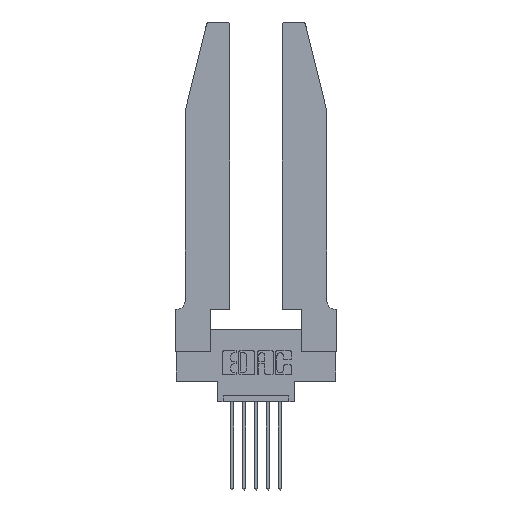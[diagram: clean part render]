
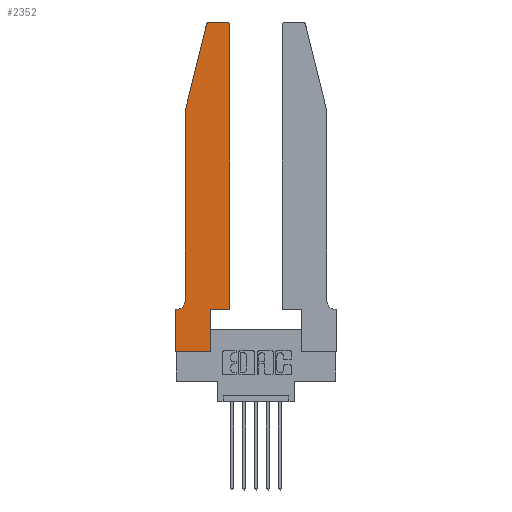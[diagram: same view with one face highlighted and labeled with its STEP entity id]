
A CAD part, top view. The second image highlights one B-rep face of the part: STEP entity #2352.
In plain terms, the highlighted planar face has unit normal (0, 0, 1).
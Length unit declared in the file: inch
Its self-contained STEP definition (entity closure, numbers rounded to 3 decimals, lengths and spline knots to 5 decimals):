
#86 = VERTEX_POINT ( 'NONE', #11882 ) ;
#117 = VECTOR ( 'NONE', #6942, 39.37008 ) ;
#277 = CARTESIAN_POINT ( 'NONE',  ( 0.284, 2.72, 0.37 ) ) ;
#532 = DIRECTION ( 'NONE',  ( 0., 1., 0. ) ) ;
#563 = VECTOR ( 'NONE', #11464, 39.37008 ) ;
#651 = EDGE_CURVE ( 'NONE', #5297, #6075, #4653, .T. ) ;
#719 = CARTESIAN_POINT ( 'NONE',  ( 0.25487, 2.72718, 0.37 ) ) ;
#742 = CARTESIAN_POINT ( 'NONE',  ( 0.0755, 2., 0.37 ) ) ;
#791 = LINE ( 'NONE', #742, #117 ) ;
#1119 = DIRECTION ( 'NONE',  ( -0.239, -0.971, 0. ) ) ;
#1229 = VERTEX_POINT ( 'NONE', #7699 ) ;
#1370 = LINE ( 'NONE', #12494, #563 ) ;
#1377 = CARTESIAN_POINT ( 'NONE',  ( 0., 0., 0.37 ) ) ;
#1384 = VERTEX_POINT ( 'NONE', #13593 ) ;
#1536 = AXIS2_PLACEMENT_3D ( 'NONE', #4381, #11823, #5419 ) ;
#1684 = CIRCLE ( 'NONE', #10323, 0.03 ) ;
#1970 = DIRECTION ( 'NONE',  ( 0., 1., 0. ) ) ;
#2149 = ORIENTED_EDGE ( 'NONE', *, *, #11321, .T. ) ;
#2274 = CARTESIAN_POINT ( 'NONE',  ( 0.0055, 0.35, 0.37 ) ) ;
#2352 = ADVANCED_FACE ( 'NONE', ( #10021 ), #7145, .T. ) ;
#2370 = DIRECTION ( 'NONE',  ( 1., 0., 0. ) ) ;
#2582 = VECTOR ( 'NONE', #1970, 39.37008 ) ;
#2630 = ORIENTED_EDGE ( 'NONE', *, *, #651, .T. ) ;
#2699 = VECTOR ( 'NONE', #1119, 39.37008 ) ;
#2728 = VERTEX_POINT ( 'NONE', #719 ) ;
#2963 = DIRECTION ( 'NONE',  ( 1., 0., 0. ) ) ;
#3282 = EDGE_CURVE ( 'NONE', #1384, #10411, #4582, .T. ) ;
#3318 = DIRECTION ( 'NONE',  ( 0., -1., 0. ) ) ;
#3495 = ORIENTED_EDGE ( 'NONE', *, *, #11349, .T. ) ;
#3652 = CIRCLE ( 'NONE', #4557, 0.03 ) ;
#3903 = VERTEX_POINT ( 'NONE', #12029 ) ;
#4160 = ORIENTED_EDGE ( 'NONE', *, *, #5319, .T. ) ;
#4203 = CARTESIAN_POINT ( 'NONE',  ( 0.0755, 0.35, 0.37 ) ) ;
#4381 = CARTESIAN_POINT ( 'NONE',  ( 0.0055, 0.42, 0.37 ) ) ;
#4391 = VECTOR ( 'NONE', #2963, 39.37008 ) ;
#4557 = AXIS2_PLACEMENT_3D ( 'NONE', #10787, #9686, #8837 ) ;
#4582 = LINE ( 'NONE', #5097, #2582 ) ;
#4653 = LINE ( 'NONE', #8917, #7781 ) ;
#5025 = DIRECTION ( 'NONE',  ( 1., 0., 0. ) ) ;
#5097 = CARTESIAN_POINT ( 'NONE',  ( 0.4505, 0.35, 0.37 ) ) ;
#5227 = EDGE_CURVE ( 'NONE', #2728, #3903, #9280, .T. ) ;
#5297 = VERTEX_POINT ( 'NONE', #11549 ) ;
#5319 = EDGE_CURVE ( 'NONE', #8497, #5297, #1370, .T. ) ;
#5395 = EDGE_CURVE ( 'NONE', #7365, #2728, #1684, .T. ) ;
#5419 = DIRECTION ( 'NONE',  ( -1., 0., 0. ) ) ;
#5600 = CARTESIAN_POINT ( 'NONE',  ( 0.4205, 2.75, 0.37 ) ) ;
#6006 = AXIS2_PLACEMENT_3D ( 'NONE', #12528, #7280, #5025 ) ;
#6075 = VERTEX_POINT ( 'NONE', #11300 ) ;
#6126 = CARTESIAN_POINT ( 'NONE',  ( 0.0755, 2., 0.37 ) ) ;
#6325 = ORIENTED_EDGE ( 'NONE', *, *, #12403, .T. ) ;
#6474 = EDGE_CURVE ( 'NONE', #86, #6538, #10070, .T. ) ;
#6538 = VERTEX_POINT ( 'NONE', #2274 ) ;
#6814 = EDGE_CURVE ( 'NONE', #10411, #6964, #3652, .T. ) ;
#6942 = DIRECTION ( 'NONE',  ( 0., -1., 0. ) ) ;
#6964 = VERTEX_POINT ( 'NONE', #5600 ) ;
#7145 = PLANE ( 'NONE',  #6006 ) ;
#7280 = DIRECTION ( 'NONE',  ( 0., 0., 1. ) ) ;
#7365 = VERTEX_POINT ( 'NONE', #12676 ) ;
#7471 = CARTESIAN_POINT ( 'NONE',  ( 0.4505, 2.72, 0.37 ) ) ;
#7496 = ORIENTED_EDGE ( 'NONE', *, *, #5395, .T. ) ;
#7500 = EDGE_LOOP ( 'NONE', ( #3495, #7496, #9881, #10154, #12679, #11388, #2149, #4160, #2630, #6325, #7884, #12615 ) ) ;
#7699 = CARTESIAN_POINT ( 'NONE',  ( 0., 0.35, 0.37 ) ) ;
#7720 = LINE ( 'NONE', #12756, #12978 ) ;
#7781 = VECTOR ( 'NONE', #532, 39.37008 ) ;
#7884 = ORIENTED_EDGE ( 'NONE', *, *, #3282, .T. ) ;
#8497 = VERTEX_POINT ( 'NONE', #9855 ) ;
#8668 = DIRECTION ( 'NONE',  ( -1., 0., 0. ) ) ;
#8704 = DIRECTION ( 'NONE',  ( 0., 0., 1. ) ) ;
#8837 = DIRECTION ( 'NONE',  ( 1., 0., 0. ) ) ;
#8917 = CARTESIAN_POINT ( 'NONE',  ( 0.2865, 0.35, 0.37 ) ) ;
#9280 = LINE ( 'NONE', #6126, #2699 ) ;
#9686 = DIRECTION ( 'NONE',  ( 0., 0., 1. ) ) ;
#9855 = CARTESIAN_POINT ( 'NONE',  ( 0., 0., 0.37 ) ) ;
#9881 = ORIENTED_EDGE ( 'NONE', *, *, #5227, .T. ) ;
#10021 = FACE_OUTER_BOUND ( 'NONE', #7500, .T. ) ;
#10070 = CIRCLE ( 'NONE', #1536, 0.07 ) ;
#10127 = LINE ( 'NONE', #12502, #4391 ) ;
#10154 = ORIENTED_EDGE ( 'NONE', *, *, #11557, .T. ) ;
#10323 = AXIS2_PLACEMENT_3D ( 'NONE', #277, #8704, #2370 ) ;
#10409 = EDGE_CURVE ( 'NONE', #6538, #1229, #11009, .T. ) ;
#10411 = VERTEX_POINT ( 'NONE', #7471 ) ;
#10758 = DIRECTION ( 'NONE',  ( -1., 0., 0. ) ) ;
#10787 = CARTESIAN_POINT ( 'NONE',  ( 0.4205, 2.72, 0.37 ) ) ;
#11009 = LINE ( 'NONE', #4203, #13336 ) ;
#11300 = CARTESIAN_POINT ( 'NONE',  ( 0.2865, 0.35, 0.37 ) ) ;
#11321 = EDGE_CURVE ( 'NONE', #1229, #8497, #13144, .T. ) ;
#11349 = EDGE_CURVE ( 'NONE', #6964, #7365, #7720, .T. ) ;
#11388 = ORIENTED_EDGE ( 'NONE', *, *, #10409, .T. ) ;
#11464 = DIRECTION ( 'NONE',  ( 1., 0., 0. ) ) ;
#11549 = CARTESIAN_POINT ( 'NONE',  ( 0.2865, 0., 0.37 ) ) ;
#11557 = EDGE_CURVE ( 'NONE', #3903, #86, #791, .T. ) ;
#11823 = DIRECTION ( 'NONE',  ( 0., 0., -1. ) ) ;
#11882 = CARTESIAN_POINT ( 'NONE',  ( 0.0755, 0.42, 0.37 ) ) ;
#12029 = CARTESIAN_POINT ( 'NONE',  ( 0.0755, 2., 0.37 ) ) ;
#12403 = EDGE_CURVE ( 'NONE', #6075, #1384, #10127, .T. ) ;
#12494 = CARTESIAN_POINT ( 'NONE',  ( 0., 0., 0.37 ) ) ;
#12502 = CARTESIAN_POINT ( 'NONE',  ( 0.4505, 0.35, 0.37 ) ) ;
#12528 = CARTESIAN_POINT ( 'NONE',  ( 0., 0.35, 0.37 ) ) ;
#12615 = ORIENTED_EDGE ( 'NONE', *, *, #6814, .T. ) ;
#12676 = CARTESIAN_POINT ( 'NONE',  ( 0.284, 2.75, 0.37 ) ) ;
#12679 = ORIENTED_EDGE ( 'NONE', *, *, #6474, .T. ) ;
#12756 = CARTESIAN_POINT ( 'NONE',  ( 0.2605, 2.75, 0.37 ) ) ;
#12817 = VECTOR ( 'NONE', #3318, 39.37008 ) ;
#12978 = VECTOR ( 'NONE', #8668, 39.37008 ) ;
#13144 = LINE ( 'NONE', #1377, #12817 ) ;
#13336 = VECTOR ( 'NONE', #10758, 39.37008 ) ;
#13593 = CARTESIAN_POINT ( 'NONE',  ( 0.4505, 0.35, 0.37 ) ) ;
